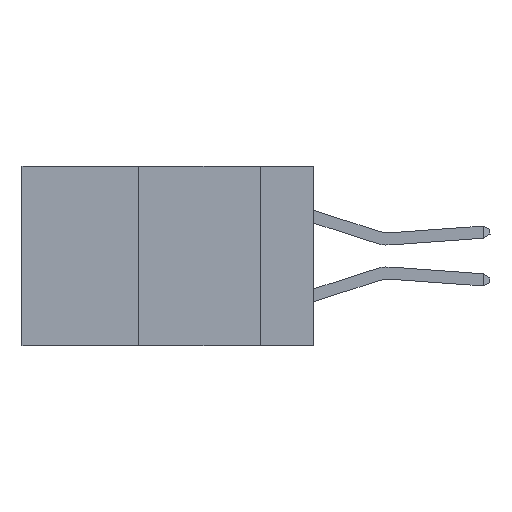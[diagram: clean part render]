
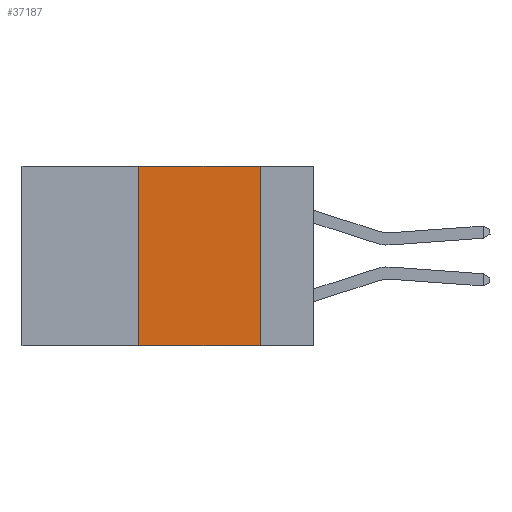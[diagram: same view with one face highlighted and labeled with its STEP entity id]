
A CAD part, left-side view. The second image highlights one B-rep face of the part: STEP entity #37187.
In plain terms, the highlighted planar face has unit normal (-1, 0, 0).
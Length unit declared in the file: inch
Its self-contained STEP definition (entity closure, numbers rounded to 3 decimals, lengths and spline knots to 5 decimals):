
#103 = PLANE ( 'NONE',  #8132 ) ;
#775 = DIRECTION ( 'NONE',  ( 0., 0., -1. ) ) ;
#1192 = VECTOR ( 'NONE', #775, 39.37008 ) ;
#1930 = VERTEX_POINT ( 'NONE', #17816 ) ;
#3426 = VERTEX_POINT ( 'NONE', #16804 ) ;
#3906 = CARTESIAN_POINT ( 'NONE',  ( 0., 0.36, 0. ) ) ;
#4522 = CARTESIAN_POINT ( 'NONE',  ( 0., 0.11, 0. ) ) ;
#6113 = VERTEX_POINT ( 'NONE', #38040 ) ;
#6659 = CARTESIAN_POINT ( 'NONE',  ( 0., 0.6, -0.37 ) ) ;
#6902 = VECTOR ( 'NONE', #27791, 39.37008 ) ;
#8132 = AXIS2_PLACEMENT_3D ( 'NONE', #12116, #35486, #8582 ) ;
#8582 = DIRECTION ( 'NONE',  ( 0., 0., -1. ) ) ;
#9069 = EDGE_LOOP ( 'NONE', ( #26239, #18411, #12695, #33870 ) ) ;
#12116 = CARTESIAN_POINT ( 'NONE',  ( 0., 0.6, 0. ) ) ;
#12695 = ORIENTED_EDGE ( 'NONE', *, *, #33306, .F. ) ;
#15072 = VERTEX_POINT ( 'NONE', #20626 ) ;
#16804 = CARTESIAN_POINT ( 'NONE',  ( 0., 0.36, 0. ) ) ;
#17816 = CARTESIAN_POINT ( 'NONE',  ( 0., 0.11, 0. ) ) ;
#18411 = ORIENTED_EDGE ( 'NONE', *, *, #37828, .F. ) ;
#18934 = LINE ( 'NONE', #36604, #6902 ) ;
#20626 = CARTESIAN_POINT ( 'NONE',  ( 0., 0.11, -0.37 ) ) ;
#20823 = LINE ( 'NONE', #6659, #24130 ) ;
#24130 = VECTOR ( 'NONE', #35743, 39.37008 ) ;
#26239 = ORIENTED_EDGE ( 'NONE', *, *, #36508, .F. ) ;
#27066 = FACE_OUTER_BOUND ( 'NONE', #9069, .T. ) ;
#27791 = DIRECTION ( 'NONE',  ( 0., -1., 0. ) ) ;
#27892 = DIRECTION ( 'NONE',  ( 0., 0., 1. ) ) ;
#29151 = EDGE_CURVE ( 'NONE', #6113, #15072, #20823, .T. ) ;
#30509 = VECTOR ( 'NONE', #27892, 39.37008 ) ;
#30817 = LINE ( 'NONE', #3906, #30509 ) ;
#30853 = LINE ( 'NONE', #4522, #1192 ) ;
#33306 = EDGE_CURVE ( 'NONE', #6113, #3426, #30817, .T. ) ;
#33870 = ORIENTED_EDGE ( 'NONE', *, *, #29151, .T. ) ;
#35486 = DIRECTION ( 'NONE',  ( 1., 0., 0. ) ) ;
#35743 = DIRECTION ( 'NONE',  ( 0., -1., 0. ) ) ;
#36508 = EDGE_CURVE ( 'NONE', #1930, #15072, #30853, .T. ) ;
#36604 = CARTESIAN_POINT ( 'NONE',  ( 0., 0.6, 0. ) ) ;
#37187 = ADVANCED_FACE ( 'NONE', ( #27066 ), #103, .F. ) ;
#37828 = EDGE_CURVE ( 'NONE', #3426, #1930, #18934, .T. ) ;
#38040 = CARTESIAN_POINT ( 'NONE',  ( 0., 0.36, -0.37 ) ) ;
